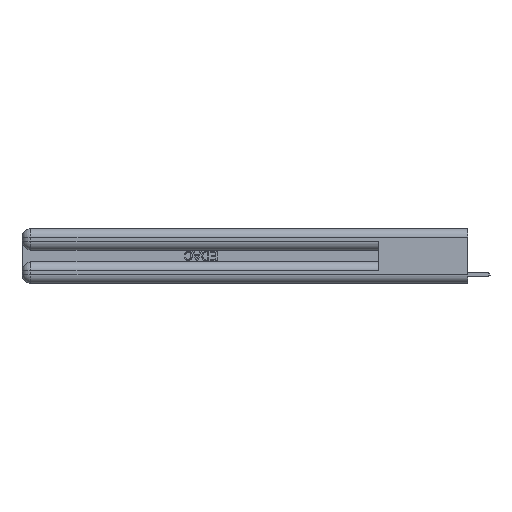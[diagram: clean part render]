
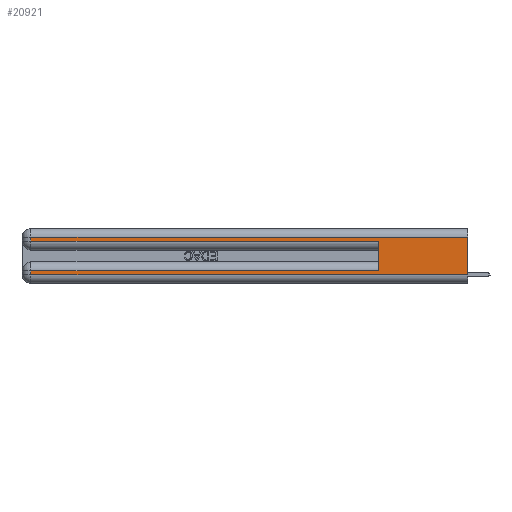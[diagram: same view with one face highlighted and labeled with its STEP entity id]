
A CAD part, left-side view. The second image highlights one B-rep face of the part: STEP entity #20921.
In plain terms, the highlighted planar face has unit normal (-1, 0, 0).
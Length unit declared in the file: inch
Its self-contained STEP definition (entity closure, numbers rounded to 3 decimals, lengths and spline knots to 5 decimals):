
#398 = EDGE_CURVE ( 'NONE', #17611, #22096, #5303, .T. ) ;
#644 = CARTESIAN_POINT ( 'NONE',  ( 0., 0.6, 0.085 ) ) ;
#2279 = DIRECTION ( 'NONE',  ( 0., 0., -1. ) ) ;
#2299 = VERTEX_POINT ( 'NONE', #644 ) ;
#3106 = LINE ( 'NONE', #14642, #30373 ) ;
#3261 = PLANE ( 'NONE',  #24352 ) ;
#3291 = EDGE_CURVE ( 'NONE', #28805, #27150, #27231, .T. ) ;
#3586 = CARTESIAN_POINT ( 'NONE',  ( 0., 2.94, 0.31 ) ) ;
#4847 = VERTEX_POINT ( 'NONE', #13735 ) ;
#5303 = LINE ( 'NONE', #29126, #7007 ) ;
#7007 = VECTOR ( 'NONE', #2279, 39.37008 ) ;
#8180 = FACE_OUTER_BOUND ( 'NONE', #12681, .T. ) ;
#8185 = CARTESIAN_POINT ( 'NONE',  ( 0., 0., 0.31 ) ) ;
#8413 = CARTESIAN_POINT ( 'NONE',  ( 0., 2.94, 0.37 ) ) ;
#9369 = EDGE_CURVE ( 'NONE', #2299, #4847, #22685, .T. ) ;
#9384 = VECTOR ( 'NONE', #15708, 39.37008 ) ;
#10358 = ORIENTED_EDGE ( 'NONE', *, *, #12989, .T. ) ;
#10515 = ORIENTED_EDGE ( 'NONE', *, *, #24313, .T. ) ;
#10558 = LINE ( 'NONE', #15281, #25956 ) ;
#10685 = CARTESIAN_POINT ( 'NONE',  ( 0., 0., 0.37 ) ) ;
#10993 = CARTESIAN_POINT ( 'NONE',  ( 0., 2.94, 0.06 ) ) ;
#11341 = VECTOR ( 'NONE', #20078, 39.37008 ) ;
#12011 = LINE ( 'NONE', #8185, #30637 ) ;
#12681 = EDGE_LOOP ( 'NONE', ( #30738, #10358, #25503, #23983, #12966, #21552, #16761, #10515 ) ) ;
#12889 = DIRECTION ( 'NONE',  ( 0., 0., 1. ) ) ;
#12966 = ORIENTED_EDGE ( 'NONE', *, *, #9369, .F. ) ;
#12989 = EDGE_CURVE ( 'NONE', #17153, #28805, #12011, .T. ) ;
#13735 = CARTESIAN_POINT ( 'NONE',  ( 0., 0.6, 0.285 ) ) ;
#14642 = CARTESIAN_POINT ( 'NONE',  ( 0., 0., 0.285 ) ) ;
#15237 = CARTESIAN_POINT ( 'NONE',  ( 0., 0., 0.37 ) ) ;
#15281 = CARTESIAN_POINT ( 'NONE',  ( 0., 0., 0.06 ) ) ;
#15391 = LINE ( 'NONE', #15237, #9384 ) ;
#15708 = DIRECTION ( 'NONE',  ( 0., 0., -1. ) ) ;
#16183 = DIRECTION ( 'NONE',  ( 0., 1., 0. ) ) ;
#16761 = ORIENTED_EDGE ( 'NONE', *, *, #398, .T. ) ;
#17049 = DIRECTION ( 'NONE',  ( 0., 1., 0. ) ) ;
#17153 = VERTEX_POINT ( 'NONE', #26235 ) ;
#17611 = VERTEX_POINT ( 'NONE', #28564 ) ;
#17814 = DIRECTION ( 'NONE',  ( 0., -1., 0. ) ) ;
#18026 = VERTEX_POINT ( 'NONE', #28994 ) ;
#20078 = DIRECTION ( 'NONE',  ( 0., 0., -1. ) ) ;
#20148 = CARTESIAN_POINT ( 'NONE',  ( 0., 0.6, 0.145 ) ) ;
#20295 = DIRECTION ( 'NONE',  ( 0., 0., -1. ) ) ;
#20921 = ADVANCED_FACE ( 'NONE', ( #8180 ), #3261, .F. ) ;
#21552 = ORIENTED_EDGE ( 'NONE', *, *, #24820, .T. ) ;
#22008 = EDGE_CURVE ( 'NONE', #27150, #4847, #3106, .T. ) ;
#22096 = VERTEX_POINT ( 'NONE', #10993 ) ;
#22378 = DIRECTION ( 'NONE',  ( 0., -1., 0. ) ) ;
#22482 = VECTOR ( 'NONE', #16183, 39.37008 ) ;
#22685 = LINE ( 'NONE', #20148, #23798 ) ;
#23798 = VECTOR ( 'NONE', #12889, 39.37008 ) ;
#23983 = ORIENTED_EDGE ( 'NONE', *, *, #22008, .T. ) ;
#24313 = EDGE_CURVE ( 'NONE', #22096, #18026, #10558, .T. ) ;
#24352 = AXIS2_PLACEMENT_3D ( 'NONE', #10685, #25216, #20295 ) ;
#24651 = EDGE_CURVE ( 'NONE', #17153, #18026, #15391, .T. ) ;
#24820 = EDGE_CURVE ( 'NONE', #2299, #17611, #25988, .T. ) ;
#25216 = DIRECTION ( 'NONE',  ( 1., 0., 0. ) ) ;
#25503 = ORIENTED_EDGE ( 'NONE', *, *, #3291, .T. ) ;
#25956 = VECTOR ( 'NONE', #17814, 39.37008 ) ;
#25988 = LINE ( 'NONE', #27892, #22482 ) ;
#26235 = CARTESIAN_POINT ( 'NONE',  ( 0., 0., 0.31 ) ) ;
#27150 = VERTEX_POINT ( 'NONE', #29679 ) ;
#27231 = LINE ( 'NONE', #8413, #11341 ) ;
#27892 = CARTESIAN_POINT ( 'NONE',  ( 0., 0., 0.085 ) ) ;
#28564 = CARTESIAN_POINT ( 'NONE',  ( 0., 2.94, 0.085 ) ) ;
#28805 = VERTEX_POINT ( 'NONE', #3586 ) ;
#28994 = CARTESIAN_POINT ( 'NONE',  ( 0., 0., 0.06 ) ) ;
#29126 = CARTESIAN_POINT ( 'NONE',  ( 0., 2.94, 0.37 ) ) ;
#29679 = CARTESIAN_POINT ( 'NONE',  ( 0., 2.94, 0.285 ) ) ;
#30373 = VECTOR ( 'NONE', #22378, 39.37008 ) ;
#30637 = VECTOR ( 'NONE', #17049, 39.37008 ) ;
#30738 = ORIENTED_EDGE ( 'NONE', *, *, #24651, .F. ) ;
